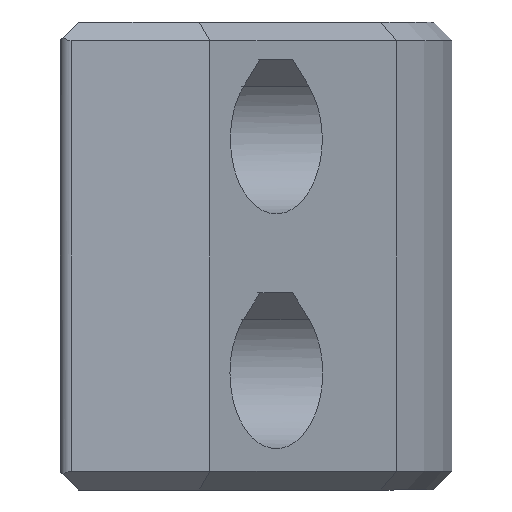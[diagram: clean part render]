
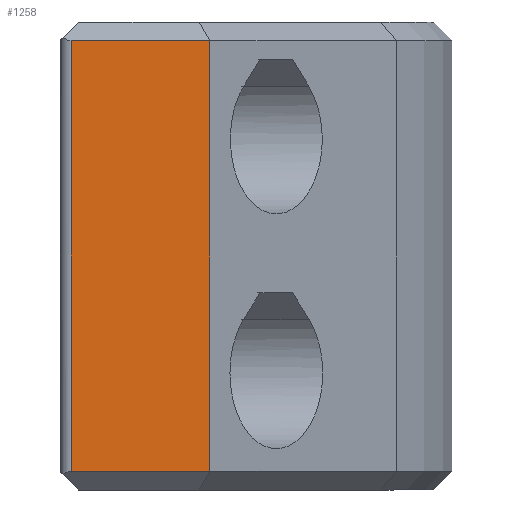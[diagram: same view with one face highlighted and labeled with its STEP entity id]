
A CAD part, front view. The second image highlights one B-rep face of the part: STEP entity #1258.
In plain terms, the highlighted planar face has unit normal (0, -1, 0).
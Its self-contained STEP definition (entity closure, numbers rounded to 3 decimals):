
#79=PLANE('',#1367);
#140=FACE_OUTER_BOUND('',#216,.T.);
#216=EDGE_LOOP('',(#979,#980,#981,#982));
#281=LINE('',#1839,#413);
#296=LINE('',#1940,#428);
#314=LINE('',#1987,#446);
#322=LINE('',#2006,#454);
#413=VECTOR('',#1469,10.);
#428=VECTOR('',#1524,10.);
#446=VECTOR('',#1568,10.);
#454=VECTOR('',#1582,10.);
#565=VERTEX_POINT('',#1836);
#566=VERTEX_POINT('',#1838);
#588=VERTEX_POINT('',#1939);
#604=VERTEX_POINT('',#1986);
#688=EDGE_CURVE('',#565,#566,#281,.T.);
#721=EDGE_CURVE('',#566,#588,#296,.T.);
#745=EDGE_CURVE('',#604,#588,#314,.T.);
#755=EDGE_CURVE('',#604,#565,#322,.T.);
#979=ORIENTED_EDGE('',*,*,#688,.F.);
#980=ORIENTED_EDGE('',*,*,#755,.F.);
#981=ORIENTED_EDGE('',*,*,#745,.T.);
#982=ORIENTED_EDGE('',*,*,#721,.F.);
#1258=ADVANCED_FACE('',(#140),#79,.T.);
#1367=AXIS2_PLACEMENT_3D('',#2005,#1580,#1581);
#1469=DIRECTION('',(0.,0.,1.));
#1524=DIRECTION('',(1.,0.,0.));
#1568=DIRECTION('',(0.,0.,1.));
#1580=DIRECTION('center_axis',(0.,-1.,0.));
#1581=DIRECTION('ref_axis',(1.,0.,0.));
#1582=DIRECTION('',(-1.,0.,0.));
#1836=CARTESIAN_POINT('',(91.971,-27.079,1.));
#1838=CARTESIAN_POINT('',(91.971,-27.079,24.));
#1839=CARTESIAN_POINT('',(91.971,-27.079,23.346));
#1939=CARTESIAN_POINT('',(99.371,-27.079,24.));
#1940=CARTESIAN_POINT('',(83.603,-27.079,24.));
#1986=CARTESIAN_POINT('',(99.371,-27.079,1.));
#1987=CARTESIAN_POINT('',(99.371,-27.079,0.));
#2005=CARTESIAN_POINT('Origin',(84.371,-27.079,0.));
#2006=CARTESIAN_POINT('',(64.678,-27.079,1.));
